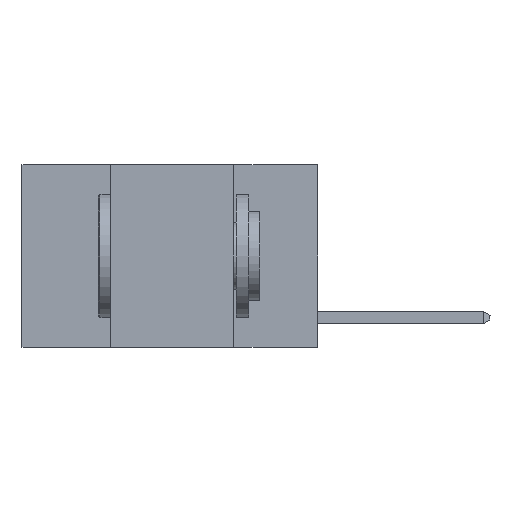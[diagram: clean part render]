
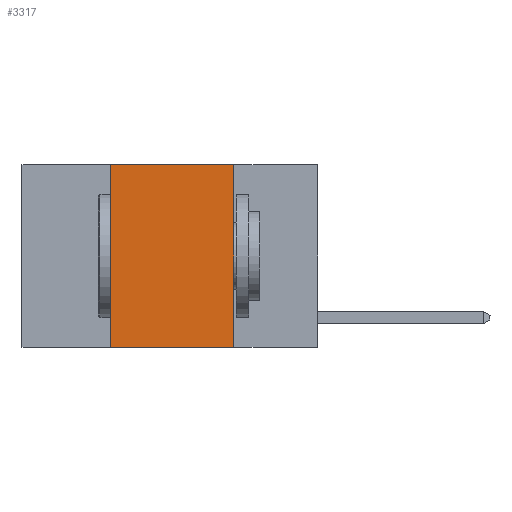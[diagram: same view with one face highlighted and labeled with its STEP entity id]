
A CAD part, left-side view. The second image highlights one B-rep face of the part: STEP entity #3317.
In plain terms, the highlighted planar face has unit normal (-1, 0, 0).
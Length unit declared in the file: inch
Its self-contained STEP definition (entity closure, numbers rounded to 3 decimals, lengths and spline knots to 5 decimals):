
#154 = DIRECTION ( 'NONE',  ( 0., -1., 0. ) ) ;
#450 = LINE ( 'NONE', #7758, #2069 ) ;
#743 = CARTESIAN_POINT ( 'NONE',  ( 0., 0.17, 0. ) ) ;
#825 = CARTESIAN_POINT ( 'NONE',  ( 0., 0.42, -0.37 ) ) ;
#1709 = ORIENTED_EDGE ( 'NONE', *, *, #4214, .F. ) ;
#1817 = DIRECTION ( 'NONE',  ( 0., -1., 0. ) ) ;
#1869 = LINE ( 'NONE', #9270, #9626 ) ;
#1959 = CARTESIAN_POINT ( 'NONE',  ( 0., 0.17, -0.37 ) ) ;
#2069 = VECTOR ( 'NONE', #5698, 39.37008 ) ;
#2304 = ORIENTED_EDGE ( 'NONE', *, *, #9249, .F. ) ;
#2351 = VECTOR ( 'NONE', #1817, 39.37008 ) ;
#3044 = CARTESIAN_POINT ( 'NONE',  ( 0., 0.42, 0. ) ) ;
#3085 = VERTEX_POINT ( 'NONE', #3044 ) ;
#3317 = ADVANCED_FACE ( 'NONE', ( #8879 ), #5125, .F. ) ;
#3694 = CARTESIAN_POINT ( 'NONE',  ( 0., 0.6, 0. ) ) ;
#4214 = EDGE_CURVE ( 'NONE', #7360, #3085, #450, .T. ) ;
#4272 = ORIENTED_EDGE ( 'NONE', *, *, #6691, .F. ) ;
#4449 = DIRECTION ( 'NONE',  ( 0., 0., -1. ) ) ;
#5125 = PLANE ( 'NONE',  #8536 ) ;
#5235 = VERTEX_POINT ( 'NONE', #8743 ) ;
#5261 = LINE ( 'NONE', #743, #6722 ) ;
#5698 = DIRECTION ( 'NONE',  ( 0., 0., 1. ) ) ;
#6503 = DIRECTION ( 'NONE',  ( 0., 0., -1. ) ) ;
#6547 = CARTESIAN_POINT ( 'NONE',  ( 0., 0.6, 0. ) ) ;
#6570 = VERTEX_POINT ( 'NONE', #1959 ) ;
#6691 = EDGE_CURVE ( 'NONE', #5235, #6570, #5261, .T. ) ;
#6722 = VECTOR ( 'NONE', #4449, 39.37008 ) ;
#7199 = ORIENTED_EDGE ( 'NONE', *, *, #9293, .T. ) ;
#7360 = VERTEX_POINT ( 'NONE', #825 ) ;
#7583 = EDGE_LOOP ( 'NONE', ( #4272, #2304, #1709, #7199 ) ) ;
#7758 = CARTESIAN_POINT ( 'NONE',  ( 0., 0.42, 0. ) ) ;
#8536 = AXIS2_PLACEMENT_3D ( 'NONE', #6547, #8781, #6503 ) ;
#8743 = CARTESIAN_POINT ( 'NONE',  ( 0., 0.17, 0. ) ) ;
#8781 = DIRECTION ( 'NONE',  ( 1., 0., 0. ) ) ;
#8879 = FACE_OUTER_BOUND ( 'NONE', #7583, .T. ) ;
#8938 = LINE ( 'NONE', #3694, #2351 ) ;
#9249 = EDGE_CURVE ( 'NONE', #3085, #5235, #8938, .T. ) ;
#9270 = CARTESIAN_POINT ( 'NONE',  ( 0., 0.6, -0.37 ) ) ;
#9293 = EDGE_CURVE ( 'NONE', #7360, #6570, #1869, .T. ) ;
#9626 = VECTOR ( 'NONE', #154, 39.37008 ) ;
